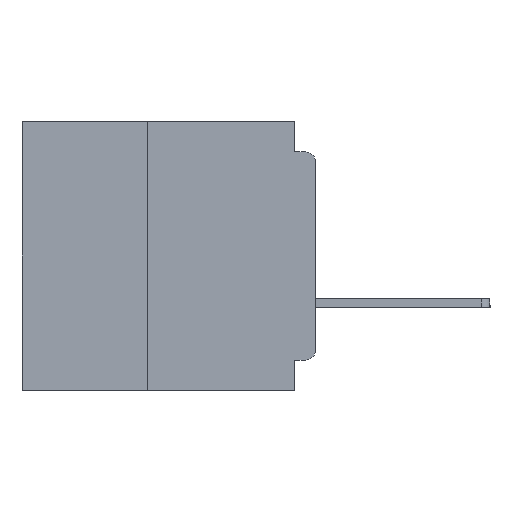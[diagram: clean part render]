
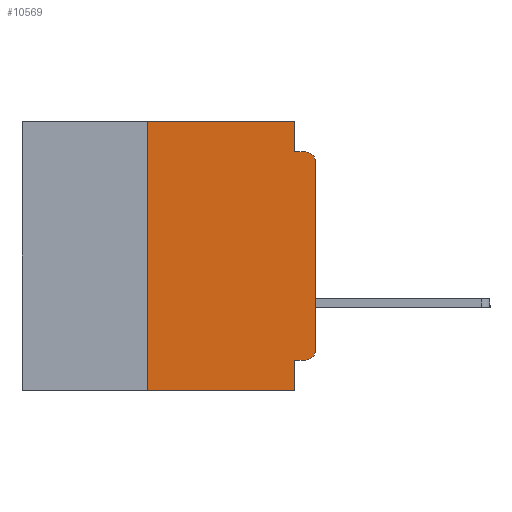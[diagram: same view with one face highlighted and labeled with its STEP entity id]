
A CAD part, left-side view. The second image highlights one B-rep face of the part: STEP entity #10569.
In plain terms, the highlighted planar face has unit normal (-1, 0, 0).
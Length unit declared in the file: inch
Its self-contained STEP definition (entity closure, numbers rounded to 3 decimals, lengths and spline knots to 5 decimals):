
#627 = ORIENTED_EDGE ( 'NONE', *, *, #3984, .F. ) ;
#849 = EDGE_CURVE ( 'NONE', #28801, #26143, #30289, .T. ) ;
#898 = AXIS2_PLACEMENT_3D ( 'NONE', #33536, #15913, #23571 ) ;
#1205 = VECTOR ( 'NONE', #13338, 39.37008 ) ;
#1767 = VERTEX_POINT ( 'NONE', #1785 ) ;
#1785 = CARTESIAN_POINT ( 'NONE',  ( 0., 0.031, -0.045 ) ) ;
#2391 = EDGE_CURVE ( 'NONE', #16396, #35376, #31512, .T. ) ;
#2807 = CARTESIAN_POINT ( 'NONE',  ( 0., 0., -0.06 ) ) ;
#2891 = CARTESIAN_POINT ( 'NONE',  ( 0., 0., -0.355 ) ) ;
#3064 = EDGE_CURVE ( 'NONE', #35376, #28801, #23043, .T. ) ;
#3431 = LINE ( 'NONE', #9201, #17692 ) ;
#3984 = EDGE_CURVE ( 'NONE', #14606, #25366, #3431, .T. ) ;
#4149 = EDGE_CURVE ( 'NONE', #5065, #25366, #35009, .T. ) ;
#4407 = EDGE_CURVE ( 'NONE', #5556, #6912, #18544, .T. ) ;
#4755 = VECTOR ( 'NONE', #27154, 39.37008 ) ;
#4882 = DIRECTION ( 'NONE',  ( 1., 0., 0. ) ) ;
#5065 = VERTEX_POINT ( 'NONE', #14240 ) ;
#5168 = VECTOR ( 'NONE', #16897, 39.37008 ) ;
#5199 = DIRECTION ( 'NONE',  ( 0., -1., 0. ) ) ;
#5513 = AXIS2_PLACEMENT_3D ( 'NONE', #26191, #26181, #26145 ) ;
#5556 = VERTEX_POINT ( 'NONE', #16448 ) ;
#5747 = DIRECTION ( 'NONE',  ( 0., 1., 0. ) ) ;
#6174 = DIRECTION ( 'NONE',  ( 0., 0., -1. ) ) ;
#6191 = LINE ( 'NONE', #33710, #12894 ) ;
#6436 = CARTESIAN_POINT ( 'NONE',  ( 0., 0.25, -0.4 ) ) ;
#6912 = VERTEX_POINT ( 'NONE', #15564 ) ;
#7466 = CARTESIAN_POINT ( 'NONE',  ( 0., 0.031, -0.355 ) ) ;
#8580 = ORIENTED_EDGE ( 'NONE', *, *, #849, .T. ) ;
#9201 = CARTESIAN_POINT ( 'NONE',  ( 0., 0.031, -0.4 ) ) ;
#9260 = EDGE_CURVE ( 'NONE', #6912, #1767, #15980, .T. ) ;
#9290 = DIRECTION ( 'NONE',  ( 0., 0., 1. ) ) ;
#9417 = CARTESIAN_POINT ( 'NONE',  ( 0., 0.015, -0.045 ) ) ;
#10569 = ADVANCED_FACE ( 'NONE', ( #31005 ), #35980, .F. ) ;
#11224 = ORIENTED_EDGE ( 'NONE', *, *, #3064, .T. ) ;
#11696 = VECTOR ( 'NONE', #5747, 39.37008 ) ;
#12894 = VECTOR ( 'NONE', #5199, 39.37008 ) ;
#13119 = ORIENTED_EDGE ( 'NONE', *, *, #4149, .T. ) ;
#13208 = CARTESIAN_POINT ( 'NONE',  ( 0., 0., 0. ) ) ;
#13338 = DIRECTION ( 'NONE',  ( 0., 0., 1. ) ) ;
#13357 = CARTESIAN_POINT ( 'NONE',  ( 0., 0.437, 0. ) ) ;
#14240 = CARTESIAN_POINT ( 'NONE',  ( 0., 0.25, -0.4 ) ) ;
#14606 = VERTEX_POINT ( 'NONE', #7466 ) ;
#15564 = CARTESIAN_POINT ( 'NONE',  ( 0., 0.031, 0. ) ) ;
#15913 = DIRECTION ( 'NONE',  ( -1., 0., 0. ) ) ;
#15980 = LINE ( 'NONE', #31728, #31125 ) ;
#16041 = EDGE_CURVE ( 'NONE', #16396, #14606, #34401, .T. ) ;
#16396 = VERTEX_POINT ( 'NONE', #35703 ) ;
#16448 = CARTESIAN_POINT ( 'NONE',  ( 0., 0.25, 0. ) ) ;
#16897 = DIRECTION ( 'NONE',  ( 0., -1., 0. ) ) ;
#17692 = VECTOR ( 'NONE', #26402, 39.37008 ) ;
#17902 = EDGE_CURVE ( 'NONE', #1767, #26143, #6191, .T. ) ;
#18166 = EDGE_CURVE ( 'NONE', #5065, #5556, #27571, .T. ) ;
#18544 = LINE ( 'NONE', #31100, #5168 ) ;
#18829 = ORIENTED_EDGE ( 'NONE', *, *, #17902, .F. ) ;
#23043 = LINE ( 'NONE', #13208, #1205 ) ;
#23367 = ORIENTED_EDGE ( 'NONE', *, *, #16041, .F. ) ;
#23571 = DIRECTION ( 'NONE',  ( 0., 0., -1. ) ) ;
#24800 = DIRECTION ( 'NONE',  ( 0., 0., -1. ) ) ;
#25214 = AXIS2_PLACEMENT_3D ( 'NONE', #13357, #4882, #24800 ) ;
#25366 = VERTEX_POINT ( 'NONE', #28643 ) ;
#26143 = VERTEX_POINT ( 'NONE', #9417 ) ;
#26145 = DIRECTION ( 'NONE',  ( 0., 0., -1. ) ) ;
#26181 = DIRECTION ( 'NONE',  ( -1., 0., 0. ) ) ;
#26191 = CARTESIAN_POINT ( 'NONE',  ( 0., 0.015, -0.34 ) ) ;
#26402 = DIRECTION ( 'NONE',  ( 0., 0., -1. ) ) ;
#27154 = DIRECTION ( 'NONE',  ( 0., -1., 0. ) ) ;
#27571 = LINE ( 'NONE', #6436, #28450 ) ;
#28450 = VECTOR ( 'NONE', #9290, 39.37008 ) ;
#28643 = CARTESIAN_POINT ( 'NONE',  ( 0., 0.031, -0.4 ) ) ;
#28801 = VERTEX_POINT ( 'NONE', #2807 ) ;
#30018 = ORIENTED_EDGE ( 'NONE', *, *, #4407, .F. ) ;
#30289 = CIRCLE ( 'NONE', #898, 0.015 ) ;
#30874 = EDGE_LOOP ( 'NONE', ( #11224, #8580, #18829, #33975, #30018, #32289, #13119, #627, #23367, #31406 ) ) ;
#31005 = FACE_OUTER_BOUND ( 'NONE', #30874, .T. ) ;
#31100 = CARTESIAN_POINT ( 'NONE',  ( 0., 0.437, 0. ) ) ;
#31125 = VECTOR ( 'NONE', #6174, 39.37008 ) ;
#31406 = ORIENTED_EDGE ( 'NONE', *, *, #2391, .T. ) ;
#31512 = CIRCLE ( 'NONE', #5513, 0.015 ) ;
#31728 = CARTESIAN_POINT ( 'NONE',  ( 0., 0.031, 0. ) ) ;
#32289 = ORIENTED_EDGE ( 'NONE', *, *, #18166, .F. ) ;
#33536 = CARTESIAN_POINT ( 'NONE',  ( 0., 0.015, -0.06 ) ) ;
#33643 = CARTESIAN_POINT ( 'NONE',  ( 0., 0., -0.34 ) ) ;
#33710 = CARTESIAN_POINT ( 'NONE',  ( 0., 0., -0.045 ) ) ;
#33975 = ORIENTED_EDGE ( 'NONE', *, *, #9260, .F. ) ;
#34401 = LINE ( 'NONE', #2891, #11696 ) ;
#35009 = LINE ( 'NONE', #35562, #4755 ) ;
#35376 = VERTEX_POINT ( 'NONE', #33643 ) ;
#35562 = CARTESIAN_POINT ( 'NONE',  ( 0., 0.437, -0.4 ) ) ;
#35703 = CARTESIAN_POINT ( 'NONE',  ( 0., 0.015, -0.355 ) ) ;
#35980 = PLANE ( 'NONE',  #25214 ) ;
